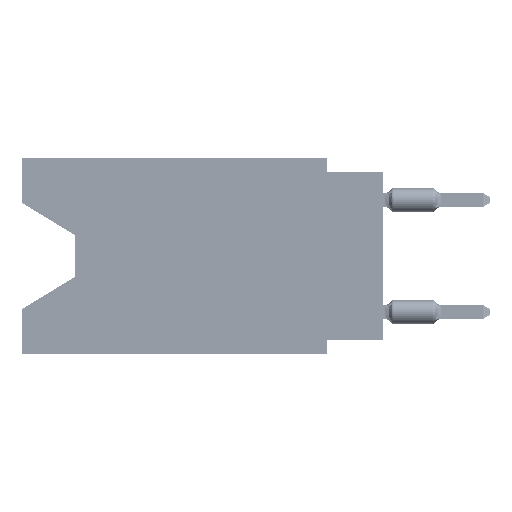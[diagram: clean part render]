
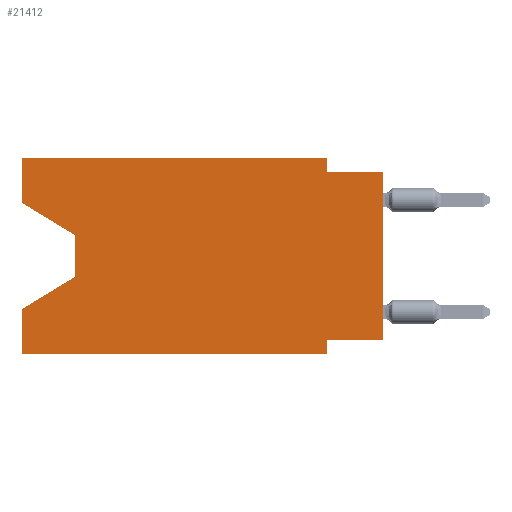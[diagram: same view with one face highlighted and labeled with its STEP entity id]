
A CAD part, left-side view. The second image highlights one B-rep face of the part: STEP entity #21412.
In plain terms, the highlighted planar face has unit normal (-1, 0, 0).
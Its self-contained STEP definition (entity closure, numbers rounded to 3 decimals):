
#600 = CARTESIAN_POINT ( 'NONE',  ( 0., 0., -8.255 ) ) ;
#880 = ORIENTED_EDGE ( 'NONE', *, *, #8380, .T. ) ;
#2360 = CARTESIAN_POINT ( 'NONE',  ( 0., 0., 0. ) ) ;
#3465 = VERTEX_POINT ( 'NONE', #14236 ) ;
#3822 = EDGE_CURVE ( 'NONE', #45614, #68509, #27894, .T. ) ;
#4621 = VERTEX_POINT ( 'NONE', #19011 ) ;
#5343 = EDGE_CURVE ( 'NONE', #55541, #78090, #76453, .T. ) ;
#5368 = ORIENTED_EDGE ( 'NONE', *, *, #20762, .T. ) ;
#5446 = CARTESIAN_POINT ( 'NONE',  ( 0., 16.383, -8.89 ) ) ;
#5899 = EDGE_CURVE ( 'NONE', #8141, #50016, #20862, .T. ) ;
#6075 = CARTESIAN_POINT ( 'NONE',  ( 0., 16.383, -2.038 ) ) ;
#8141 = VERTEX_POINT ( 'NONE', #20680 ) ;
#8380 = EDGE_CURVE ( 'NONE', #45614, #8141, #55528, .T. ) ;
#9105 = DIRECTION ( 'NONE',  ( 0., 0., 1. ) ) ;
#9749 = CARTESIAN_POINT ( 'NONE',  ( 0., 16.383, 0. ) ) ;
#10332 = VECTOR ( 'NONE', #59554, 1000. ) ;
#10839 = DIRECTION ( 'NONE',  ( 1., 0., 0. ) ) ;
#11219 = PLANE ( 'NONE',  #68844 ) ;
#12638 = LINE ( 'NONE', #36095, #51085 ) ;
#12890 = LINE ( 'NONE', #600, #78459 ) ;
#13088 = CARTESIAN_POINT ( 'NONE',  ( 0., 0., -0.635 ) ) ;
#13151 = ORIENTED_EDGE ( 'NONE', *, *, #29479, .F. ) ;
#14236 = CARTESIAN_POINT ( 'NONE',  ( 0., 16.383, -6.852 ) ) ;
#15215 = DIRECTION ( 'NONE',  ( 0., 0., 1. ) ) ;
#15281 = DIRECTION ( 'NONE',  ( 0., 0., -1. ) ) ;
#17881 = CARTESIAN_POINT ( 'NONE',  ( 0., 2.54, 0. ) ) ;
#19011 = CARTESIAN_POINT ( 'NONE',  ( 0., 0., -0.635 ) ) ;
#19044 = LINE ( 'NONE', #13088, #27804 ) ;
#20680 = CARTESIAN_POINT ( 'NONE',  ( 0., 13.97, -3.505 ) ) ;
#20762 = EDGE_CURVE ( 'NONE', #22934, #78090, #59852, .T. ) ;
#20862 = LINE ( 'NONE', #63347, #33450 ) ;
#21412 = ADVANCED_FACE ( 'NONE', ( #46566 ), #11219, .F. ) ;
#21950 = ORIENTED_EDGE ( 'NONE', *, *, #5343, .F. ) ;
#22062 = CARTESIAN_POINT ( 'NONE',  ( 0., 2.54, -8.89 ) ) ;
#22823 = LINE ( 'NONE', #9749, #35306 ) ;
#22934 = VERTEX_POINT ( 'NONE', #59830 ) ;
#23214 = DIRECTION ( 'NONE',  ( 0., 0., 1. ) ) ;
#23490 = CARTESIAN_POINT ( 'NONE',  ( 0., 13.97, -5.385 ) ) ;
#23949 = VECTOR ( 'NONE', #60720, 1000. ) ;
#25787 = DIRECTION ( 'NONE',  ( 0., -1., 0. ) ) ;
#26838 = EDGE_LOOP ( 'NONE', ( #880, #52936, #70231, #13151, #5368, #21950, #51739, #32842, #48526, #53753, #38525, #65736 ) ) ;
#27804 = VECTOR ( 'NONE', #25787, 1000. ) ;
#27894 = LINE ( 'NONE', #69222, #34546 ) ;
#29479 = EDGE_CURVE ( 'NONE', #22934, #3465, #22823, .T. ) ;
#29652 = DIRECTION ( 'NONE',  ( 0., -1., 0. ) ) ;
#30117 = EDGE_CURVE ( 'NONE', #70704, #55541, #12890, .T. ) ;
#30535 = EDGE_CURVE ( 'NONE', #60724, #4621, #19044, .T. ) ;
#32842 = ORIENTED_EDGE ( 'NONE', *, *, #33931, .T. ) ;
#33450 = VECTOR ( 'NONE', #15281, 1000. ) ;
#33931 = EDGE_CURVE ( 'NONE', #70704, #4621, #56768, .T. ) ;
#34546 = VECTOR ( 'NONE', #15215, 1000. ) ;
#35306 = VECTOR ( 'NONE', #23214, 1000. ) ;
#36095 = CARTESIAN_POINT ( 'NONE',  ( 0., 16.383, 0. ) ) ;
#36634 = CARTESIAN_POINT ( 'NONE',  ( 0., 13.97, -5.385 ) ) ;
#38359 = CARTESIAN_POINT ( 'NONE',  ( 0., 2.54, 0. ) ) ;
#38525 = ORIENTED_EDGE ( 'NONE', *, *, #48861, .F. ) ;
#40335 = DIRECTION ( 'NONE',  ( 0., 0., -1. ) ) ;
#41857 = VECTOR ( 'NONE', #60860, 1000. ) ;
#44569 = VECTOR ( 'NONE', #9105, 1000. ) ;
#45554 = EDGE_CURVE ( 'NONE', #50016, #3465, #65669, .T. ) ;
#45614 = VERTEX_POINT ( 'NONE', #6075 ) ;
#45828 = CARTESIAN_POINT ( 'NONE',  ( 0., 0., -8.255 ) ) ;
#46566 = FACE_OUTER_BOUND ( 'NONE', #26838, .T. ) ;
#47638 = CARTESIAN_POINT ( 'NONE',  ( 0., 16.383, 0. ) ) ;
#48526 = ORIENTED_EDGE ( 'NONE', *, *, #30535, .F. ) ;
#48861 = EDGE_CURVE ( 'NONE', #68509, #71319, #12638, .T. ) ;
#49425 = DIRECTION ( 'NONE',  ( 0., 1., 0. ) ) ;
#50016 = VERTEX_POINT ( 'NONE', #23490 ) ;
#51085 = VECTOR ( 'NONE', #54742, 1000. ) ;
#51739 = ORIENTED_EDGE ( 'NONE', *, *, #30117, .F. ) ;
#52918 = CARTESIAN_POINT ( 'NONE',  ( 0., 16.383, 0. ) ) ;
#52936 = ORIENTED_EDGE ( 'NONE', *, *, #5899, .T. ) ;
#53753 = ORIENTED_EDGE ( 'NONE', *, *, #67311, .F. ) ;
#54742 = DIRECTION ( 'NONE',  ( 0., -1., 0. ) ) ;
#55528 = LINE ( 'NONE', #61490, #23949 ) ;
#55541 = VERTEX_POINT ( 'NONE', #69562 ) ;
#56768 = LINE ( 'NONE', #2360, #44569 ) ;
#56786 = CARTESIAN_POINT ( 'NONE',  ( 0., 2.54, -0.635 ) ) ;
#57499 = VECTOR ( 'NONE', #40335, 1000. ) ;
#58772 = CARTESIAN_POINT ( 'NONE',  ( 0., 2.54, -8.89 ) ) ;
#59554 = DIRECTION ( 'NONE',  ( 0., 0., -1. ) ) ;
#59830 = CARTESIAN_POINT ( 'NONE',  ( 0., 16.383, -8.89 ) ) ;
#59852 = LINE ( 'NONE', #5446, #62446 ) ;
#60720 = DIRECTION ( 'NONE',  ( 0., -0.855, -0.519 ) ) ;
#60724 = VERTEX_POINT ( 'NONE', #56786 ) ;
#60860 = DIRECTION ( 'NONE',  ( 0., 0.855, -0.519 ) ) ;
#61490 = CARTESIAN_POINT ( 'NONE',  ( 0., 16.383, -2.038 ) ) ;
#62446 = VECTOR ( 'NONE', #29652, 1000. ) ;
#63347 = CARTESIAN_POINT ( 'NONE',  ( 0., 13.97, -3.505 ) ) ;
#65127 = LINE ( 'NONE', #38359, #10332 ) ;
#65611 = DIRECTION ( 'NONE',  ( 0., 0., -1. ) ) ;
#65669 = LINE ( 'NONE', #36634, #41857 ) ;
#65736 = ORIENTED_EDGE ( 'NONE', *, *, #3822, .F. ) ;
#67311 = EDGE_CURVE ( 'NONE', #71319, #60724, #65127, .T. ) ;
#68509 = VERTEX_POINT ( 'NONE', #47638 ) ;
#68844 = AXIS2_PLACEMENT_3D ( 'NONE', #52918, #10839, #65611 ) ;
#69222 = CARTESIAN_POINT ( 'NONE',  ( 0., 16.383, 0. ) ) ;
#69562 = CARTESIAN_POINT ( 'NONE',  ( 0., 2.54, -8.255 ) ) ;
#70231 = ORIENTED_EDGE ( 'NONE', *, *, #45554, .T. ) ;
#70704 = VERTEX_POINT ( 'NONE', #45828 ) ;
#71319 = VERTEX_POINT ( 'NONE', #17881 ) ;
#76453 = LINE ( 'NONE', #22062, #57499 ) ;
#78090 = VERTEX_POINT ( 'NONE', #58772 ) ;
#78459 = VECTOR ( 'NONE', #49425, 1000. ) ;
